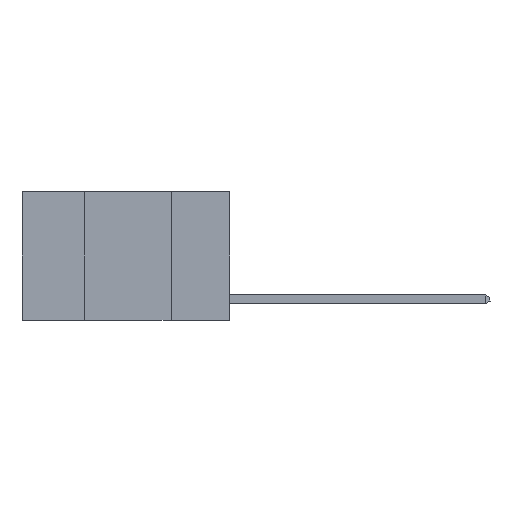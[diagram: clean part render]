
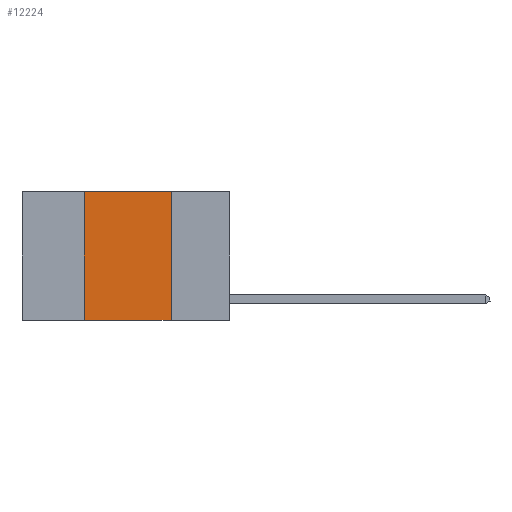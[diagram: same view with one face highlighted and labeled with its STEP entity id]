
A CAD part, left-side view. The second image highlights one B-rep face of the part: STEP entity #12224.
In plain terms, the highlighted planar face has unit normal (-1, 0, 0).
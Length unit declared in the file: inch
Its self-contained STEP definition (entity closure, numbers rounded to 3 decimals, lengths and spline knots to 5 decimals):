
#148 = LINE ( 'NONE', #17914, #7815 ) ;
#295 = VERTEX_POINT ( 'NONE', #18088 ) ;
#352 = VECTOR ( 'NONE', #944, 39.37008 ) ;
#944 = DIRECTION ( 'NONE',  ( 0., 0., 1. ) ) ;
#1821 = CARTESIAN_POINT ( 'NONE',  ( 0., 0.17, 0. ) ) ;
#1912 = DIRECTION ( 'NONE',  ( 0., -1., 0. ) ) ;
#1914 = DIRECTION ( 'NONE',  ( 0., -1., 0. ) ) ;
#2252 = ORIENTED_EDGE ( 'NONE', *, *, #11315, .F. ) ;
#2879 = VECTOR ( 'NONE', #1914, 39.37008 ) ;
#3677 = VECTOR ( 'NONE', #6274, 39.37008 ) ;
#4093 = EDGE_CURVE ( 'NONE', #12689, #8391, #148, .T. ) ;
#6274 = DIRECTION ( 'NONE',  ( 0., 0., -1. ) ) ;
#6460 = ORIENTED_EDGE ( 'NONE', *, *, #4093, .T. ) ;
#6646 = AXIS2_PLACEMENT_3D ( 'NONE', #9318, #7593, #7528 ) ;
#7528 = DIRECTION ( 'NONE',  ( 0., 0., -1. ) ) ;
#7593 = DIRECTION ( 'NONE',  ( 1., 0., 0. ) ) ;
#7670 = ORIENTED_EDGE ( 'NONE', *, *, #17066, .F. ) ;
#7791 = PLANE ( 'NONE',  #6646 ) ;
#7815 = VECTOR ( 'NONE', #1912, 39.37008 ) ;
#7820 = LINE ( 'NONE', #9501, #3677 ) ;
#8391 = VERTEX_POINT ( 'NONE', #16741 ) ;
#8761 = LINE ( 'NONE', #17622, #2879 ) ;
#9292 = EDGE_LOOP ( 'NONE', ( #7670, #12542, #2252, #6460 ) ) ;
#9318 = CARTESIAN_POINT ( 'NONE',  ( 0., 0.6, 0. ) ) ;
#9501 = CARTESIAN_POINT ( 'NONE',  ( 0., 0.17, 0. ) ) ;
#11189 = EDGE_CURVE ( 'NONE', #295, #12281, #8761, .T. ) ;
#11191 = CARTESIAN_POINT ( 'NONE',  ( 0., 0.42, 0. ) ) ;
#11315 = EDGE_CURVE ( 'NONE', #12689, #295, #19095, .T. ) ;
#12224 = ADVANCED_FACE ( 'NONE', ( #16384 ), #7791, .F. ) ;
#12281 = VERTEX_POINT ( 'NONE', #1821 ) ;
#12542 = ORIENTED_EDGE ( 'NONE', *, *, #11189, .F. ) ;
#12689 = VERTEX_POINT ( 'NONE', #15595 ) ;
#15595 = CARTESIAN_POINT ( 'NONE',  ( 0., 0.42, -0.37 ) ) ;
#16384 = FACE_OUTER_BOUND ( 'NONE', #9292, .T. ) ;
#16741 = CARTESIAN_POINT ( 'NONE',  ( 0., 0.17, -0.37 ) ) ;
#17066 = EDGE_CURVE ( 'NONE', #12281, #8391, #7820, .T. ) ;
#17622 = CARTESIAN_POINT ( 'NONE',  ( 0., 0.6, 0. ) ) ;
#17914 = CARTESIAN_POINT ( 'NONE',  ( 0., 0.6, -0.37 ) ) ;
#18088 = CARTESIAN_POINT ( 'NONE',  ( 0., 0.42, 0. ) ) ;
#19095 = LINE ( 'NONE', #11191, #352 ) ;
